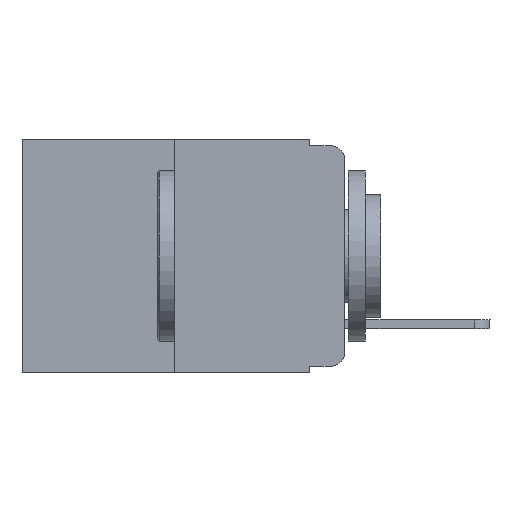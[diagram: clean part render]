
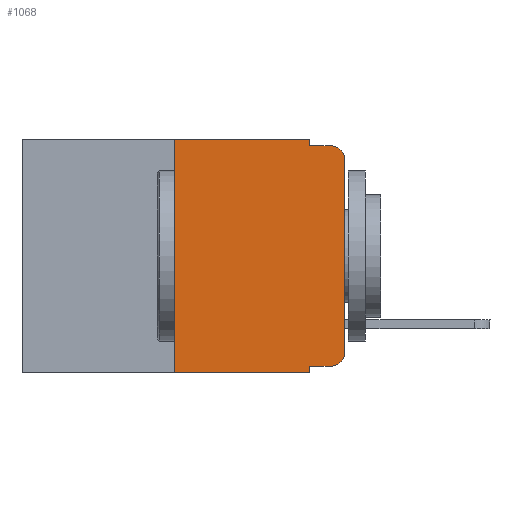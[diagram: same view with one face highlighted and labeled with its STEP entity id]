
A CAD part, left-side view. The second image highlights one B-rep face of the part: STEP entity #1068.
In plain terms, the highlighted planar face has unit normal (-1, 0, 0).
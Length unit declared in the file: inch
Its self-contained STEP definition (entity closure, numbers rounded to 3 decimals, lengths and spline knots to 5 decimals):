
#198 = ORIENTED_EDGE ( 'NONE', *, *, #414, .T. ) ;
#243 = DIRECTION ( 'NONE',  ( 0., 0., -1. ) ) ;
#414 = EDGE_CURVE ( 'NONE', #9597, #1228, #2534, .T. ) ;
#420 = LINE ( 'NONE', #1458, #8090 ) ;
#423 = CARTESIAN_POINT ( 'NONE',  ( 0., 0.051, 0. ) ) ;
#574 = EDGE_CURVE ( 'NONE', #4708, #3781, #7894, .T. ) ;
#608 = CARTESIAN_POINT ( 'NONE',  ( 0., 0., -0.313 ) ) ;
#877 = CARTESIAN_POINT ( 'NONE',  ( 0., 0.051, 0. ) ) ;
#882 = CARTESIAN_POINT ( 'NONE',  ( 0., 0.473, -0.343 ) ) ;
#939 = DIRECTION ( 'NONE',  ( 0., 0., -1. ) ) ;
#953 = LINE ( 'NONE', #3687, #4171 ) ;
#1068 = ADVANCED_FACE ( 'NONE', ( #9805 ), #7518, .F. ) ;
#1097 = AXIS2_PLACEMENT_3D ( 'NONE', #1966, #7344, #1252 ) ;
#1218 = ORIENTED_EDGE ( 'NONE', *, *, #1428, .T. ) ;
#1228 = VERTEX_POINT ( 'NONE', #608 ) ;
#1239 = DIRECTION ( 'NONE',  ( 0., 0., -1. ) ) ;
#1252 = DIRECTION ( 'NONE',  ( 0., 0., -1. ) ) ;
#1425 = LINE ( 'NONE', #877, #6631 ) ;
#1428 = EDGE_CURVE ( 'NONE', #11047, #9597, #953, .T. ) ;
#1458 = CARTESIAN_POINT ( 'NONE',  ( 0., 0.051, 0. ) ) ;
#1529 = DIRECTION ( 'NONE',  ( 0., -1., 0. ) ) ;
#1586 = ORIENTED_EDGE ( 'NONE', *, *, #7117, .F. ) ;
#1642 = DIRECTION ( 'NONE',  ( -1., 0., 0. ) ) ;
#1878 = CARTESIAN_POINT ( 'NONE',  ( 0., 0.051, -0.01 ) ) ;
#1966 = CARTESIAN_POINT ( 'NONE',  ( 0., 0.02, -0.03 ) ) ;
#2006 = VECTOR ( 'NONE', #3609, 39.37008 ) ;
#2033 = VERTEX_POINT ( 'NONE', #4699 ) ;
#2159 = VERTEX_POINT ( 'NONE', #423 ) ;
#2186 = CARTESIAN_POINT ( 'NONE',  ( 0., 0., 0. ) ) ;
#2356 = VERTEX_POINT ( 'NONE', #1878 ) ;
#2534 = CIRCLE ( 'NONE', #8352, 0.02 ) ;
#2974 = DIRECTION ( 'NONE',  ( 1., 0., 0. ) ) ;
#3202 = CARTESIAN_POINT ( 'NONE',  ( 0., 0.25, 0. ) ) ;
#3214 = CARTESIAN_POINT ( 'NONE',  ( 0., 0.02, -0.313 ) ) ;
#3390 = DIRECTION ( 'NONE',  ( 0., -1., 0. ) ) ;
#3473 = EDGE_CURVE ( 'NONE', #2356, #2033, #6243, .T. ) ;
#3481 = EDGE_CURVE ( 'NONE', #2159, #2356, #1425, .T. ) ;
#3609 = DIRECTION ( 'NONE',  ( 0., -1., 0. ) ) ;
#3687 = CARTESIAN_POINT ( 'NONE',  ( 0., 0.051, -0.333 ) ) ;
#3781 = VERTEX_POINT ( 'NONE', #3202 ) ;
#4030 = ORIENTED_EDGE ( 'NONE', *, *, #5577, .F. ) ;
#4171 = VECTOR ( 'NONE', #6137, 39.37008 ) ;
#4285 = CARTESIAN_POINT ( 'NONE',  ( 0., 0.051, -0.333 ) ) ;
#4356 = ORIENTED_EDGE ( 'NONE', *, *, #8136, .T. ) ;
#4507 = CARTESIAN_POINT ( 'NONE',  ( 0., 0.051, -0.343 ) ) ;
#4699 = CARTESIAN_POINT ( 'NONE',  ( 0., 0.02, -0.01 ) ) ;
#4708 = VERTEX_POINT ( 'NONE', #8873 ) ;
#4979 = VECTOR ( 'NONE', #1529, 39.37008 ) ;
#5115 = EDGE_LOOP ( 'NONE', ( #7327, #6400, #5468, #8876, #4030, #10603, #4356, #1586, #1218, #198 ) ) ;
#5300 = EDGE_CURVE ( 'NONE', #1228, #7143, #7400, .T. ) ;
#5468 = ORIENTED_EDGE ( 'NONE', *, *, #3473, .F. ) ;
#5577 = EDGE_CURVE ( 'NONE', #3781, #2159, #7895, .T. ) ;
#5686 = DIRECTION ( 'NONE',  ( 0., 0., 1. ) ) ;
#5832 = VECTOR ( 'NONE', #5686, 39.37008 ) ;
#6076 = CARTESIAN_POINT ( 'NONE',  ( 0., 0.25, 0. ) ) ;
#6137 = DIRECTION ( 'NONE',  ( 0., -1., 0. ) ) ;
#6243 = LINE ( 'NONE', #10536, #4979 ) ;
#6385 = CARTESIAN_POINT ( 'NONE',  ( 0., 0.02, -0.333 ) ) ;
#6400 = ORIENTED_EDGE ( 'NONE', *, *, #6501, .T. ) ;
#6501 = EDGE_CURVE ( 'NONE', #7143, #2033, #9498, .T. ) ;
#6631 = VECTOR ( 'NONE', #939, 39.37008 ) ;
#6714 = CARTESIAN_POINT ( 'NONE',  ( 0., 0., -0.03 ) ) ;
#7010 = LINE ( 'NONE', #882, #7233 ) ;
#7117 = EDGE_CURVE ( 'NONE', #11047, #8812, #420, .T. ) ;
#7143 = VERTEX_POINT ( 'NONE', #6714 ) ;
#7233 = VECTOR ( 'NONE', #3390, 39.37008 ) ;
#7316 = CARTESIAN_POINT ( 'NONE',  ( 0., 0.473, 0. ) ) ;
#7327 = ORIENTED_EDGE ( 'NONE', *, *, #5300, .T. ) ;
#7344 = DIRECTION ( 'NONE',  ( -1., 0., 0. ) ) ;
#7400 = LINE ( 'NONE', #2186, #5832 ) ;
#7518 = PLANE ( 'NONE',  #9797 ) ;
#7777 = VECTOR ( 'NONE', #9525, 39.37008 ) ;
#7894 = LINE ( 'NONE', #6076, #7777 ) ;
#7895 = LINE ( 'NONE', #10540, #2006 ) ;
#8090 = VECTOR ( 'NONE', #1239, 39.37008 ) ;
#8136 = EDGE_CURVE ( 'NONE', #4708, #8812, #7010, .T. ) ;
#8352 = AXIS2_PLACEMENT_3D ( 'NONE', #3214, #1642, #11011 ) ;
#8812 = VERTEX_POINT ( 'NONE', #4507 ) ;
#8873 = CARTESIAN_POINT ( 'NONE',  ( 0., 0.25, -0.343 ) ) ;
#8876 = ORIENTED_EDGE ( 'NONE', *, *, #3481, .F. ) ;
#9498 = CIRCLE ( 'NONE', #1097, 0.02 ) ;
#9525 = DIRECTION ( 'NONE',  ( 0., 0., 1. ) ) ;
#9597 = VERTEX_POINT ( 'NONE', #6385 ) ;
#9797 = AXIS2_PLACEMENT_3D ( 'NONE', #7316, #2974, #243 ) ;
#9805 = FACE_OUTER_BOUND ( 'NONE', #5115, .T. ) ;
#10536 = CARTESIAN_POINT ( 'NONE',  ( 0., 0.051, -0.01 ) ) ;
#10540 = CARTESIAN_POINT ( 'NONE',  ( 0., 0.473, 0. ) ) ;
#10603 = ORIENTED_EDGE ( 'NONE', *, *, #574, .F. ) ;
#11011 = DIRECTION ( 'NONE',  ( 0., 0., -1. ) ) ;
#11047 = VERTEX_POINT ( 'NONE', #4285 ) ;
